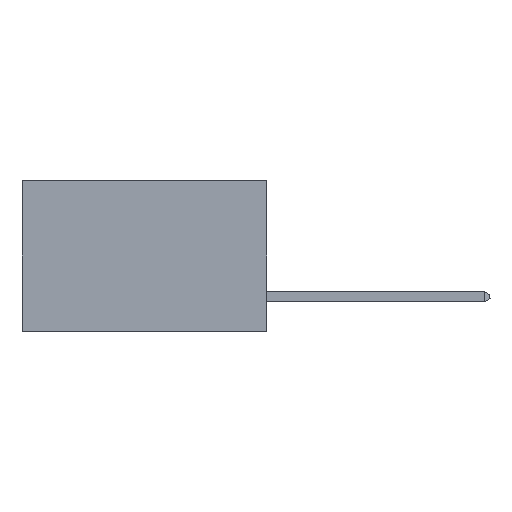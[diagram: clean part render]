
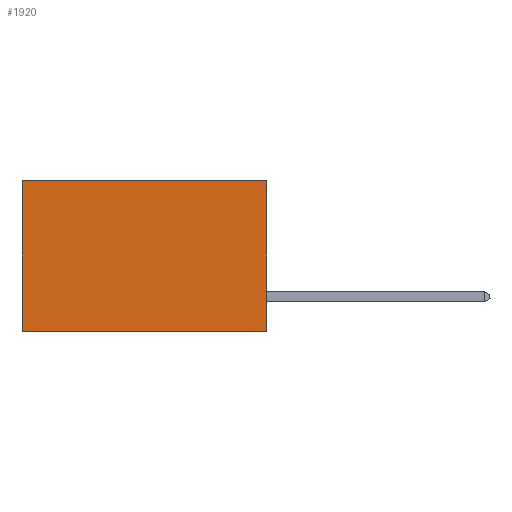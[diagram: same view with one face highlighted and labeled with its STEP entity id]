
A CAD part, left-side view. The second image highlights one B-rep face of the part: STEP entity #1920.
In plain terms, the highlighted planar face has unit normal (-1, 0, 0).
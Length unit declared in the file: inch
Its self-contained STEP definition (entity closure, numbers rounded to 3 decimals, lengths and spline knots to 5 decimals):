
#1353 = LINE ( 'NONE', #6341, #9462 ) ;
#1537 = ORIENTED_EDGE ( 'NONE', *, *, #6240, .T. ) ;
#1663 = VECTOR ( 'NONE', #2608, 39.37008 ) ;
#1801 = PLANE ( 'NONE',  #10756 ) ;
#1838 = EDGE_LOOP ( 'NONE', ( #3197, #9056, #8601, #1537 ) ) ;
#1920 = ADVANCED_FACE ( 'NONE', ( #2597 ), #1801, .F. ) ;
#2597 = FACE_OUTER_BOUND ( 'NONE', #1838, .T. ) ;
#2608 = DIRECTION ( 'NONE',  ( 0., 1., 0. ) ) ;
#2896 = DIRECTION ( 'NONE',  ( 1., 0., 0. ) ) ;
#2956 = LINE ( 'NONE', #11371, #6693 ) ;
#2985 = EDGE_CURVE ( 'NONE', #10126, #7974, #7620, .T. ) ;
#3068 = VERTEX_POINT ( 'NONE', #3577 ) ;
#3197 = ORIENTED_EDGE ( 'NONE', *, *, #2985, .T. ) ;
#3539 = DIRECTION ( 'NONE',  ( 0., 0., -1. ) ) ;
#3577 = CARTESIAN_POINT ( 'NONE',  ( 0.2875, 0., 0. ) ) ;
#4067 = LINE ( 'NONE', #9703, #1663 ) ;
#5662 = CARTESIAN_POINT ( 'NONE',  ( 0.2875, 0.6, 0. ) ) ;
#6123 = DIRECTION ( 'NONE',  ( 0., 1., 0. ) ) ;
#6187 = CARTESIAN_POINT ( 'NONE',  ( 0.2875, 0.6, 0. ) ) ;
#6240 = EDGE_CURVE ( 'NONE', #3068, #10126, #4067, .T. ) ;
#6275 = EDGE_CURVE ( 'NONE', #3068, #9031, #1353, .T. ) ;
#6341 = CARTESIAN_POINT ( 'NONE',  ( 0.2875, 0., 0. ) ) ;
#6504 = VECTOR ( 'NONE', #3539, 39.37008 ) ;
#6693 = VECTOR ( 'NONE', #6123, 39.37008 ) ;
#7189 = DIRECTION ( 'NONE',  ( 0., 0., -1. ) ) ;
#7620 = LINE ( 'NONE', #5662, #6504 ) ;
#7974 = VERTEX_POINT ( 'NONE', #9916 ) ;
#8207 = DIRECTION ( 'NONE',  ( 0., 0., -1. ) ) ;
#8601 = ORIENTED_EDGE ( 'NONE', *, *, #6275, .F. ) ;
#8957 = CARTESIAN_POINT ( 'NONE',  ( 0.2875, 0., -0.37 ) ) ;
#9031 = VERTEX_POINT ( 'NONE', #8957 ) ;
#9056 = ORIENTED_EDGE ( 'NONE', *, *, #10738, .F. ) ;
#9462 = VECTOR ( 'NONE', #7189, 39.37008 ) ;
#9703 = CARTESIAN_POINT ( 'NONE',  ( 0.2875, 0., 0. ) ) ;
#9916 = CARTESIAN_POINT ( 'NONE',  ( 0.2875, 0.6, -0.37 ) ) ;
#10126 = VERTEX_POINT ( 'NONE', #6187 ) ;
#10738 = EDGE_CURVE ( 'NONE', #9031, #7974, #2956, .T. ) ;
#10756 = AXIS2_PLACEMENT_3D ( 'NONE', #11471, #2896, #8207 ) ;
#11371 = CARTESIAN_POINT ( 'NONE',  ( 0.2875, 0., -0.37 ) ) ;
#11471 = CARTESIAN_POINT ( 'NONE',  ( 0.2875, 0., 0. ) ) ;
